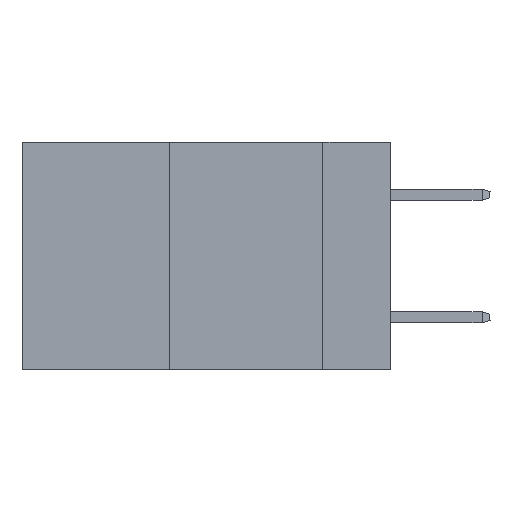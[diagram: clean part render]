
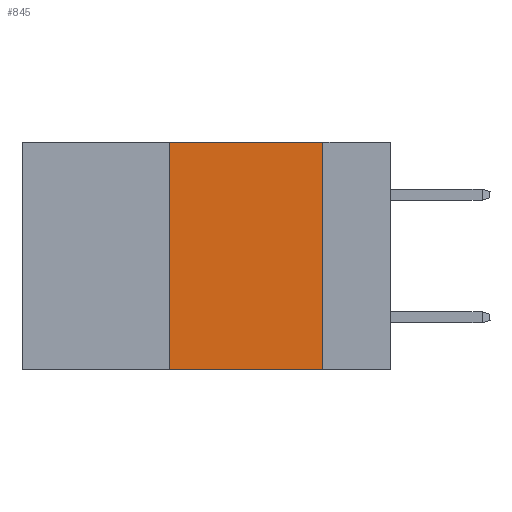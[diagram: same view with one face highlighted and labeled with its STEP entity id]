
A CAD part, left-side view. The second image highlights one B-rep face of the part: STEP entity #845.
In plain terms, the highlighted planar face has unit normal (-1, 0, 0).
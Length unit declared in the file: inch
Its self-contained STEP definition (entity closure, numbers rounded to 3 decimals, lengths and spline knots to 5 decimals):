
#355 = DIRECTION ( 'NONE',  ( 0., 0., 1. ) ) ;
#845 = ADVANCED_FACE ( 'NONE', ( #2658 ), #1972, .F. ) ;
#1972 = PLANE ( 'NONE',  #26846 ) ;
#2045 = VERTEX_POINT ( 'NONE', #19470 ) ;
#2479 = VERTEX_POINT ( 'NONE', #9916 ) ;
#2658 = FACE_OUTER_BOUND ( 'NONE', #18776, .T. ) ;
#3164 = CARTESIAN_POINT ( 'NONE',  ( 0., 0.36, -0.37 ) ) ;
#3883 = VECTOR ( 'NONE', #10123, 39.37008 ) ;
#5300 = VECTOR ( 'NONE', #25569, 39.37008 ) ;
#6138 = LINE ( 'NONE', #14679, #3883 ) ;
#6905 = CARTESIAN_POINT ( 'NONE',  ( 0., 0.36, 0. ) ) ;
#7607 = ORIENTED_EDGE ( 'NONE', *, *, #12933, .F. ) ;
#9916 = CARTESIAN_POINT ( 'NONE',  ( 0., 0.11, -0.37 ) ) ;
#10123 = DIRECTION ( 'NONE',  ( 0., -1., 0. ) ) ;
#10464 = CARTESIAN_POINT ( 'NONE',  ( 0., 0.36, 0. ) ) ;
#11385 = VERTEX_POINT ( 'NONE', #3164 ) ;
#11732 = VECTOR ( 'NONE', #20972, 39.37008 ) ;
#12500 = CARTESIAN_POINT ( 'NONE',  ( 0., 0.11, 0. ) ) ;
#12933 = EDGE_CURVE ( 'NONE', #25005, #2045, #6138, .T. ) ;
#13514 = LINE ( 'NONE', #17132, #5300 ) ;
#14679 = CARTESIAN_POINT ( 'NONE',  ( 0., 0.6, 0. ) ) ;
#14812 = LINE ( 'NONE', #10464, #25030 ) ;
#17132 = CARTESIAN_POINT ( 'NONE',  ( 0., 0.6, -0.37 ) ) ;
#18627 = ORIENTED_EDGE ( 'NONE', *, *, #26776, .T. ) ;
#18776 = EDGE_LOOP ( 'NONE', ( #23686, #7607, #24607, #18627 ) ) ;
#19470 = CARTESIAN_POINT ( 'NONE',  ( 0., 0.11, 0. ) ) ;
#20942 = CARTESIAN_POINT ( 'NONE',  ( 0., 0.6, 0. ) ) ;
#20946 = LINE ( 'NONE', #12500, #11732 ) ;
#20972 = DIRECTION ( 'NONE',  ( 0., 0., -1. ) ) ;
#22267 = EDGE_CURVE ( 'NONE', #2045, #2479, #20946, .T. ) ;
#23686 = ORIENTED_EDGE ( 'NONE', *, *, #22267, .F. ) ;
#24607 = ORIENTED_EDGE ( 'NONE', *, *, #26690, .F. ) ;
#24766 = DIRECTION ( 'NONE',  ( 1., 0., 0. ) ) ;
#25005 = VERTEX_POINT ( 'NONE', #6905 ) ;
#25030 = VECTOR ( 'NONE', #355, 39.37008 ) ;
#25569 = DIRECTION ( 'NONE',  ( 0., -1., 0. ) ) ;
#26690 = EDGE_CURVE ( 'NONE', #11385, #25005, #14812, .T. ) ;
#26776 = EDGE_CURVE ( 'NONE', #11385, #2479, #13514, .T. ) ;
#26846 = AXIS2_PLACEMENT_3D ( 'NONE', #20942, #24766, #26968 ) ;
#26968 = DIRECTION ( 'NONE',  ( 0., 0., -1. ) ) ;
